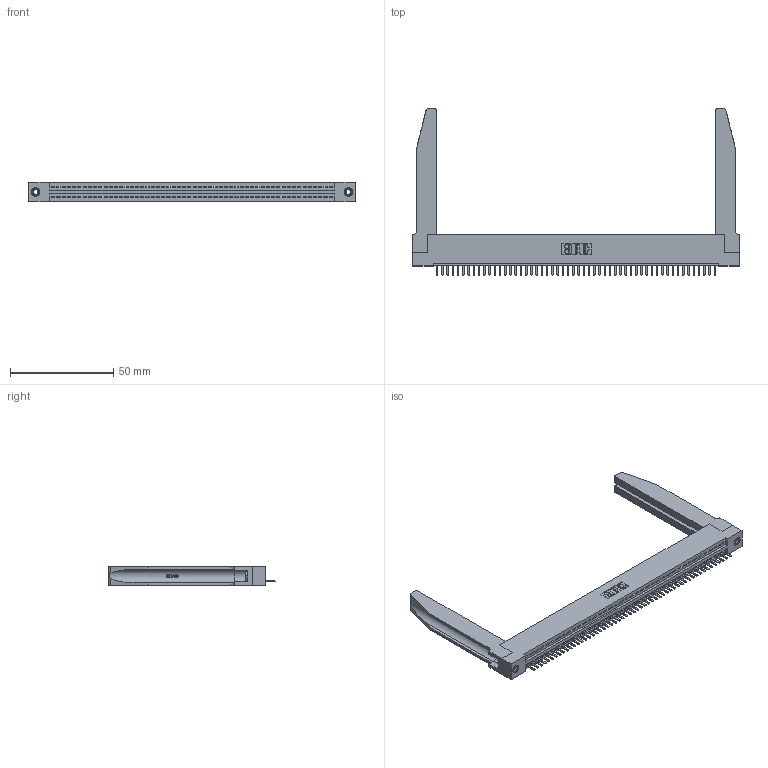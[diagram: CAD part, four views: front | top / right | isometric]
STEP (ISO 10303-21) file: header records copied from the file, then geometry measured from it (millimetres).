
FILE_DESCRIPTION (( 'STEP AP203' ), '1' );
FILE_NAME ('395-054-520-178.STEP', '2019-10-23T16:21:35', ( '' ), ( '' ), 'SwSTEP 2.0', 'SolidWorks 2016', '' );
FILE_SCHEMA (( 'CONFIG_CONTROL_DESIGN' ));
Length unit declared in the file: inch
Products named in the file (5): 345-220-078_345-220-078; 395-054-520-178; 345-292-001_345-293-120; 345 Part_Flush Mounting Lugs - 0.156 Dia-TH; 345-250-001_345-250-001-102
Assembly tree (59 placements, depth 2):
  395-054-520-178
    345 Part_Flush Mounting Lugs - 0.156 Dia-TH
    345-292-001_345-293-120  x54
    345-250-001_345-250-001-102  x2
    345-220-078_345-220-078  x2
Bounding box: 158.39 x 80.64 x 9.4 mm (x, y, z)
Volume: 22757.9 mm3; surface area: 26417.5 mm2
Topology: 59 solids, 59 shells, 3708 faces, 10885 edges, 7102 vertices
Faces by surface type: plane 2490, cylinder 1166, bspline 36, cone 12, torus 4
Entity records: 43880 total; most frequent: CARTESIAN_POINT 8509, ORIENTED_EDGE 7382, DIRECTION 6409, EDGE_CURVE 3691, VECTOR 3245, LINE 3245, VERTEX_POINT 2452, AXIS2_PLACEMENT_3D 1582
